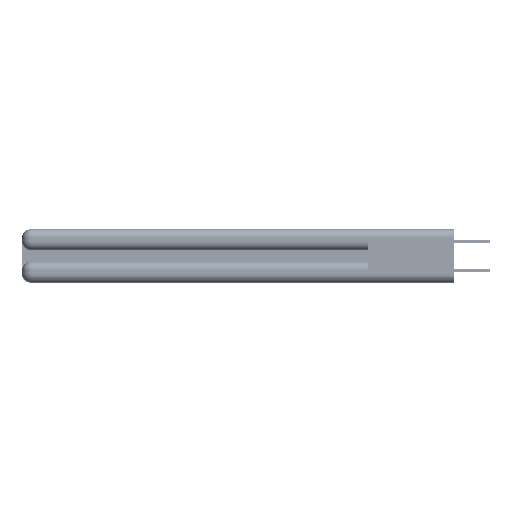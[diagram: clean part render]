
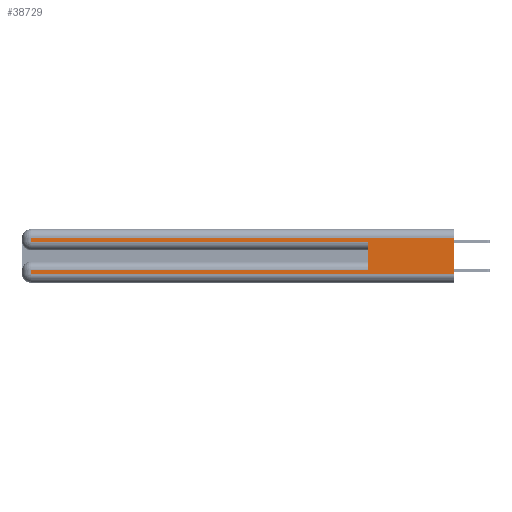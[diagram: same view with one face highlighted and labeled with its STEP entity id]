
A CAD part, left-side view. The second image highlights one B-rep face of the part: STEP entity #38729.
In plain terms, the highlighted planar face has unit normal (-1, 0, 0).
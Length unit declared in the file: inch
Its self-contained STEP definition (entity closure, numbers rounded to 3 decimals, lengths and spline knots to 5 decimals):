
#62 = ORIENTED_EDGE ( 'NONE', *, *, #45417, .T. ) ;
#471 = DIRECTION ( 'NONE',  ( 1., 0., 0. ) ) ;
#522 = LINE ( 'NONE', #18612, #45932 ) ;
#1754 = LINE ( 'NONE', #46498, #5894 ) ;
#3361 = VERTEX_POINT ( 'NONE', #43808 ) ;
#3501 = CARTESIAN_POINT ( 'NONE',  ( 0., 2.94, 0.06 ) ) ;
#3806 = CARTESIAN_POINT ( 'NONE',  ( 0., 0., 0.06 ) ) ;
#5894 = VECTOR ( 'NONE', #41891, 39.37008 ) ;
#6365 = CARTESIAN_POINT ( 'NONE',  ( 0., 0., 0.31 ) ) ;
#6485 = ORIENTED_EDGE ( 'NONE', *, *, #9704, .T. ) ;
#7214 = ORIENTED_EDGE ( 'NONE', *, *, #36387, .T. ) ;
#8232 = ORIENTED_EDGE ( 'NONE', *, *, #46776, .T. ) ;
#8627 = ORIENTED_EDGE ( 'NONE', *, *, #45596, .F. ) ;
#9402 = LINE ( 'NONE', #32067, #35518 ) ;
#9616 = CARTESIAN_POINT ( 'NONE',  ( 0., 0.6, 0.085 ) ) ;
#9704 = EDGE_CURVE ( 'NONE', #48370, #3361, #21520, .T. ) ;
#11381 = VECTOR ( 'NONE', #49412, 39.37008 ) ;
#12550 = VERTEX_POINT ( 'NONE', #3501 ) ;
#12849 = VERTEX_POINT ( 'NONE', #9616 ) ;
#14895 = EDGE_CURVE ( 'NONE', #12849, #55083, #23025, .T. ) ;
#16465 = VERTEX_POINT ( 'NONE', #3806 ) ;
#17083 = EDGE_CURVE ( 'NONE', #12849, #56340, #9402, .T. ) ;
#17147 = VECTOR ( 'NONE', #50086, 39.37008 ) ;
#18612 = CARTESIAN_POINT ( 'NONE',  ( 0., 0., 0.285 ) ) ;
#19123 = ORIENTED_EDGE ( 'NONE', *, *, #17083, .F. ) ;
#20123 = DIRECTION ( 'NONE',  ( 0., 1., 0. ) ) ;
#20585 = EDGE_LOOP ( 'NONE', ( #8627, #6485, #7214, #62, #19123, #34348, #8232, #29627 ) ) ;
#21520 = LINE ( 'NONE', #6365, #24943 ) ;
#23025 = LINE ( 'NONE', #44964, #11381 ) ;
#23835 = CARTESIAN_POINT ( 'NONE',  ( 0., 2.94, 0.285 ) ) ;
#23856 = CARTESIAN_POINT ( 'NONE',  ( 0., 2.94, 0.37 ) ) ;
#24719 = DIRECTION ( 'NONE',  ( 0., 0., -1. ) ) ;
#24943 = VECTOR ( 'NONE', #20123, 39.37008 ) ;
#27132 = CARTESIAN_POINT ( 'NONE',  ( 0., 0., 0.37 ) ) ;
#27341 = VERTEX_POINT ( 'NONE', #23835 ) ;
#29144 = CARTESIAN_POINT ( 'NONE',  ( 0., 0., 0.37 ) ) ;
#29212 = DIRECTION ( 'NONE',  ( 0., -1., 0. ) ) ;
#29325 = VECTOR ( 'NONE', #24719, 39.37008 ) ;
#29627 = ORIENTED_EDGE ( 'NONE', *, *, #39109, .T. ) ;
#32067 = CARTESIAN_POINT ( 'NONE',  ( 0., 0.6, 0.145 ) ) ;
#32962 = CARTESIAN_POINT ( 'NONE',  ( 0., 0.6, 0.285 ) ) ;
#34348 = ORIENTED_EDGE ( 'NONE', *, *, #14895, .T. ) ;
#35434 = DIRECTION ( 'NONE',  ( 0., 0., 1. ) ) ;
#35518 = VECTOR ( 'NONE', #35434, 39.37008 ) ;
#36387 = EDGE_CURVE ( 'NONE', #3361, #27341, #50919, .T. ) ;
#37228 = CARTESIAN_POINT ( 'NONE',  ( 0., 2.94, 0.085 ) ) ;
#38729 = ADVANCED_FACE ( 'NONE', ( #56332 ), #53940, .F. ) ;
#39076 = VECTOR ( 'NONE', #29212, 39.37008 ) ;
#39109 = EDGE_CURVE ( 'NONE', #12550, #16465, #40470, .T. ) ;
#40470 = LINE ( 'NONE', #55234, #39076 ) ;
#41891 = DIRECTION ( 'NONE',  ( 0., 0., -1. ) ) ;
#43182 = LINE ( 'NONE', #29144, #29325 ) ;
#43808 = CARTESIAN_POINT ( 'NONE',  ( 0., 2.94, 0.31 ) ) ;
#44494 = DIRECTION ( 'NONE',  ( 0., 0., -1. ) ) ;
#44964 = CARTESIAN_POINT ( 'NONE',  ( 0., 0., 0.085 ) ) ;
#45417 = EDGE_CURVE ( 'NONE', #27341, #56340, #522, .T. ) ;
#45596 = EDGE_CURVE ( 'NONE', #48370, #16465, #43182, .T. ) ;
#45932 = VECTOR ( 'NONE', #49440, 39.37008 ) ;
#46498 = CARTESIAN_POINT ( 'NONE',  ( 0., 2.94, 0.37 ) ) ;
#46776 = EDGE_CURVE ( 'NONE', #55083, #12550, #1754, .T. ) ;
#48370 = VERTEX_POINT ( 'NONE', #53082 ) ;
#49412 = DIRECTION ( 'NONE',  ( 0., 1., 0. ) ) ;
#49440 = DIRECTION ( 'NONE',  ( 0., -1., 0. ) ) ;
#50086 = DIRECTION ( 'NONE',  ( 0., 0., -1. ) ) ;
#50919 = LINE ( 'NONE', #23856, #17147 ) ;
#53082 = CARTESIAN_POINT ( 'NONE',  ( 0., 0., 0.31 ) ) ;
#53157 = AXIS2_PLACEMENT_3D ( 'NONE', #27132, #471, #44494 ) ;
#53940 = PLANE ( 'NONE',  #53157 ) ;
#55083 = VERTEX_POINT ( 'NONE', #37228 ) ;
#55234 = CARTESIAN_POINT ( 'NONE',  ( 0., 0., 0.06 ) ) ;
#56332 = FACE_OUTER_BOUND ( 'NONE', #20585, .T. ) ;
#56340 = VERTEX_POINT ( 'NONE', #32962 ) ;
